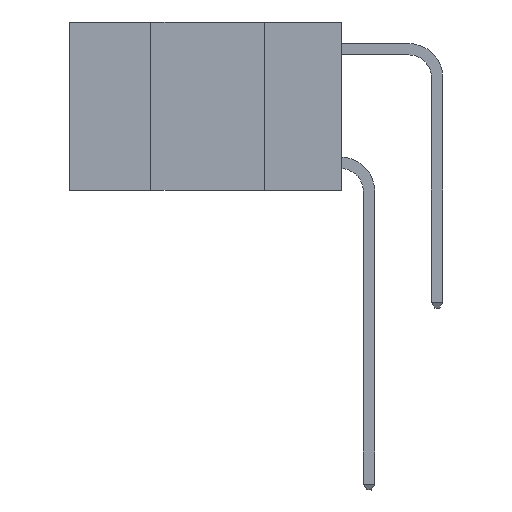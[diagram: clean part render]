
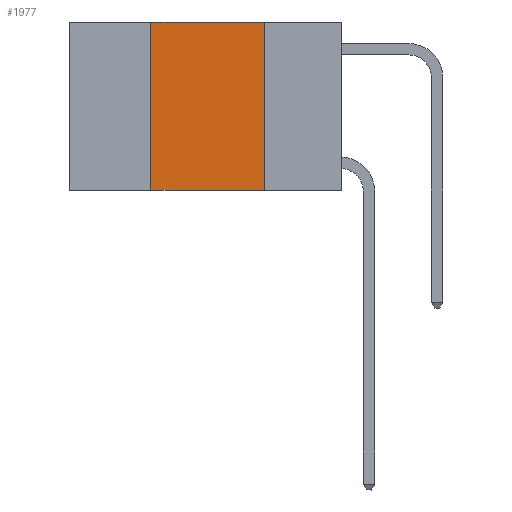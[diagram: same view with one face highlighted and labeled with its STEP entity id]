
A CAD part, left-side view. The second image highlights one B-rep face of the part: STEP entity #1977.
In plain terms, the highlighted planar face has unit normal (-1, 0, 0).
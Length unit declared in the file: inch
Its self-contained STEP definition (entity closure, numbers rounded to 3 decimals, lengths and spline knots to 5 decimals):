
#152 = CARTESIAN_POINT ( 'NONE',  ( 0., 0.42, 0. ) ) ;
#725 = ORIENTED_EDGE ( 'NONE', *, *, #6736, .F. ) ;
#1041 = VECTOR ( 'NONE', #12052, 39.37008 ) ;
#1838 = DIRECTION ( 'NONE',  ( 0., -1., 0. ) ) ;
#1862 = CARTESIAN_POINT ( 'NONE',  ( 0., 0.6, 0. ) ) ;
#1977 = ADVANCED_FACE ( 'NONE', ( #4478 ), #6326, .F. ) ;
#2497 = EDGE_LOOP ( 'NONE', ( #8400, #725, #4975, #13203 ) ) ;
#3838 = VERTEX_POINT ( 'NONE', #18655 ) ;
#4478 = FACE_OUTER_BOUND ( 'NONE', #2497, .T. ) ;
#4749 = VERTEX_POINT ( 'NONE', #9887 ) ;
#4975 = ORIENTED_EDGE ( 'NONE', *, *, #14479, .F. ) ;
#5227 = DIRECTION ( 'NONE',  ( 0., 0., -1. ) ) ;
#5620 = LINE ( 'NONE', #14985, #1041 ) ;
#6108 = CARTESIAN_POINT ( 'NONE',  ( 0., 0.6, -0.37 ) ) ;
#6326 = PLANE ( 'NONE',  #12992 ) ;
#6736 = EDGE_CURVE ( 'NONE', #17443, #3838, #15284, .T. ) ;
#7000 = LINE ( 'NONE', #6108, #14199 ) ;
#7453 = VECTOR ( 'NONE', #5227, 39.37008 ) ;
#8400 = ORIENTED_EDGE ( 'NONE', *, *, #16218, .F. ) ;
#9544 = CARTESIAN_POINT ( 'NONE',  ( 0., 0.6, 0. ) ) ;
#9887 = CARTESIAN_POINT ( 'NONE',  ( 0., 0.17, -0.37 ) ) ;
#11172 = LINE ( 'NONE', #16756, #7453 ) ;
#12052 = DIRECTION ( 'NONE',  ( 0., 0., 1. ) ) ;
#12080 = DIRECTION ( 'NONE',  ( 0., 0., -1. ) ) ;
#12992 = AXIS2_PLACEMENT_3D ( 'NONE', #1862, #18004, #12080 ) ;
#13203 = ORIENTED_EDGE ( 'NONE', *, *, #14480, .T. ) ;
#14199 = VECTOR ( 'NONE', #1838, 39.37008 ) ;
#14479 = EDGE_CURVE ( 'NONE', #16206, #17443, #5620, .T. ) ;
#14480 = EDGE_CURVE ( 'NONE', #16206, #4749, #7000, .T. ) ;
#14985 = CARTESIAN_POINT ( 'NONE',  ( 0., 0.42, 0. ) ) ;
#15047 = VECTOR ( 'NONE', #16986, 39.37008 ) ;
#15284 = LINE ( 'NONE', #9544, #15047 ) ;
#15429 = CARTESIAN_POINT ( 'NONE',  ( 0., 0.42, -0.37 ) ) ;
#16206 = VERTEX_POINT ( 'NONE', #15429 ) ;
#16218 = EDGE_CURVE ( 'NONE', #3838, #4749, #11172, .T. ) ;
#16756 = CARTESIAN_POINT ( 'NONE',  ( 0., 0.17, 0. ) ) ;
#16986 = DIRECTION ( 'NONE',  ( 0., -1., 0. ) ) ;
#17443 = VERTEX_POINT ( 'NONE', #152 ) ;
#18004 = DIRECTION ( 'NONE',  ( 1., 0., 0. ) ) ;
#18655 = CARTESIAN_POINT ( 'NONE',  ( 0., 0.17, 0. ) ) ;
